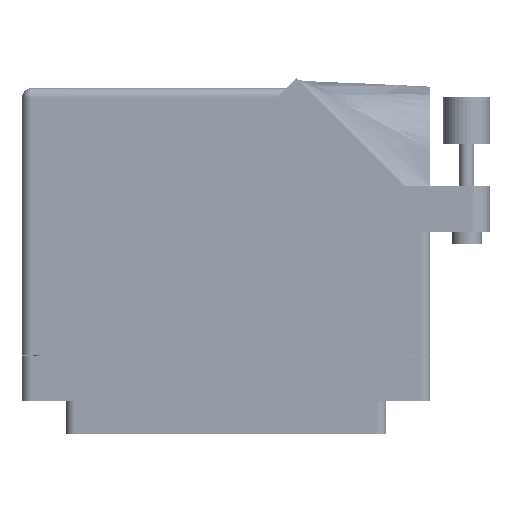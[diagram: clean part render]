
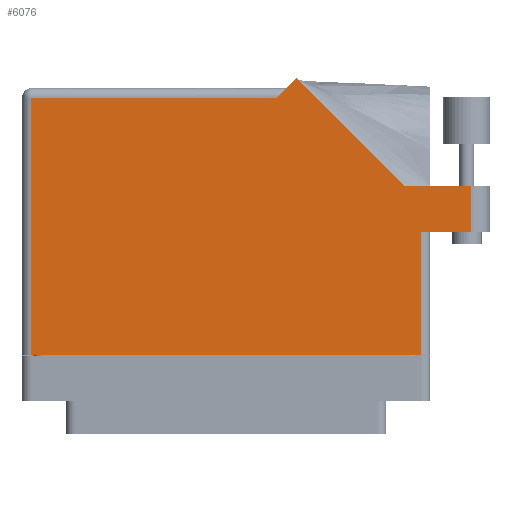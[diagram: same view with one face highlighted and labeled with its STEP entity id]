
A CAD part, front view. The second image highlights one B-rep face of the part: STEP entity #6076.
In plain terms, the highlighted face is planar.
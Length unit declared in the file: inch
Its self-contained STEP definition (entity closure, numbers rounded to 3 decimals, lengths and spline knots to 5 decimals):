
#868 = CARTESIAN_POINT ( 'NONE',  ( 1.359, 0.715, 0.617 ) ) ;
#1662 = VERTEX_POINT ( 'NONE', #10121 ) ;
#1802 = VERTEX_POINT ( 'NONE', #48628 ) ;
#1908 = VECTOR ( 'NONE', #8769, 39.37008 ) ;
#2494 = DIRECTION ( 'NONE',  ( 0., 1., 0. ) ) ;
#3832 = VECTOR ( 'NONE', #12226, 39.37008 ) ;
#4876 = CARTESIAN_POINT ( 'NONE',  ( -1.359, 1.613, 0.617 ) ) ;
#5480 = ORIENTED_EDGE ( 'NONE', *, *, #29514, .T. ) ;
#5575 = CARTESIAN_POINT ( 'NONE',  ( 1.297, 0.715, 0.617 ) ) ;
#6076 = ADVANCED_FACE ( 'NONE', ( #17635 ), #61496, .F. ) ;
#6463 = EDGE_CURVE ( 'NONE', #30711, #50482, #65937, .T. ) ;
#7562 = CARTESIAN_POINT ( 'NONE',  ( 1.297, 0.715, 0.617 ) ) ;
#8769 = DIRECTION ( 'NONE',  ( 0., 1., 0. ) ) ;
#8822 = CARTESIAN_POINT ( 'NONE',  ( 1.634, 1.022, 0.617 ) ) ;
#9809 = ORIENTED_EDGE ( 'NONE', *, *, #14939, .T. ) ;
#10024 = EDGE_CURVE ( 'NONE', #1802, #54385, #40155, .T. ) ;
#10121 = CARTESIAN_POINT ( 'NONE',  ( 0.46971, 1.74571, 0.617 ) ) ;
#10816 = CARTESIAN_POINT ( 'NONE',  ( 0.399, 1.675, 0.617 ) ) ;
#11078 = DIRECTION ( 'NONE',  ( -1., 0., 0. ) ) ;
#11191 = VECTOR ( 'NONE', #18649, 39.37008 ) ;
#12226 = DIRECTION ( 'NONE',  ( -0.707, 0.707, 0. ) ) ;
#14412 = VERTEX_POINT ( 'NONE', #29894 ) ;
#14939 = EDGE_CURVE ( 'NONE', #50482, #19580, #47428, .T. ) ;
#16135 = VECTOR ( 'NONE', #55921, 39.37008 ) ;
#17635 = FACE_OUTER_BOUND ( 'NONE', #51609, .T. ) ;
#18326 = LINE ( 'NONE', #22954, #3832 ) ;
#18385 = EDGE_CURVE ( 'NONE', #54385, #14412, #27615, .T. ) ;
#18621 = CARTESIAN_POINT ( 'NONE',  ( 1.759, 1.022, 0.617 ) ) ;
#18649 = DIRECTION ( 'NONE',  ( 0., -1., 0. ) ) ;
#19580 = VERTEX_POINT ( 'NONE', #8822 ) ;
#20605 = DIRECTION ( 'NONE',  ( 1., 0., 0. ) ) ;
#22954 = CARTESIAN_POINT ( 'NONE',  ( 1.19342, 1.022, 0.617 ) ) ;
#25347 = LINE ( 'NONE', #18621, #67749 ) ;
#26410 = LINE ( 'NONE', #4876, #32932 ) ;
#26836 = ORIENTED_EDGE ( 'NONE', *, *, #67394, .T. ) ;
#27278 = EDGE_CURVE ( 'NONE', #14412, #30711, #47818, .T. ) ;
#27615 = LINE ( 'NONE', #60590, #53027 ) ;
#29134 = CARTESIAN_POINT ( 'NONE',  ( -1.297, -0.1, 0.617 ) ) ;
#29514 = EDGE_CURVE ( 'NONE', #1662, #36642, #34059, .T. ) ;
#29646 = CARTESIAN_POINT ( 'NONE',  ( 1.634, 1.022, 0.617 ) ) ;
#29894 = CARTESIAN_POINT ( 'NONE',  ( 1.297, -0.1, 0.617 ) ) ;
#30711 = VERTEX_POINT ( 'NONE', #5575 ) ;
#32504 = ORIENTED_EDGE ( 'NONE', *, *, #41628, .T. ) ;
#32932 = VECTOR ( 'NONE', #11078, 39.37008 ) ;
#34059 = LINE ( 'NONE', #10816, #16135 ) ;
#34781 = EDGE_CURVE ( 'NONE', #64329, #1662, #18326, .T. ) ;
#35302 = DIRECTION ( 'NONE',  ( -1., 0., 0. ) ) ;
#36444 = DIRECTION ( 'NONE',  ( -1., 0., 0. ) ) ;
#36489 = ORIENTED_EDGE ( 'NONE', *, *, #10024, .T. ) ;
#36642 = VERTEX_POINT ( 'NONE', #54017 ) ;
#37693 = CARTESIAN_POINT ( 'NONE',  ( -1.297, -0.1, 0.617 ) ) ;
#38258 = CARTESIAN_POINT ( 'NONE',  ( 1.634, 0.715, 0.617 ) ) ;
#38642 = ORIENTED_EDGE ( 'NONE', *, *, #18385, .T. ) ;
#40155 = LINE ( 'NONE', #29134, #11191 ) ;
#40264 = CARTESIAN_POINT ( 'NONE',  ( -1.359, 1.675, 0.617 ) ) ;
#40407 = ORIENTED_EDGE ( 'NONE', *, *, #27278, .T. ) ;
#41628 = EDGE_CURVE ( 'NONE', #19580, #64329, #25347, .T. ) ;
#43174 = DIRECTION ( 'NONE',  ( 1., 0., 0. ) ) ;
#47428 = LINE ( 'NONE', #29646, #62671 ) ;
#47818 = LINE ( 'NONE', #7562, #1908 ) ;
#48628 = CARTESIAN_POINT ( 'NONE',  ( -1.297, 1.613, 0.617 ) ) ;
#50482 = VERTEX_POINT ( 'NONE', #38258 ) ;
#51585 = VECTOR ( 'NONE', #43174, 39.37008 ) ;
#51597 = DIRECTION ( 'NONE',  ( 0., 0., -1. ) ) ;
#51609 = EDGE_LOOP ( 'NONE', ( #55543, #9809, #32504, #52272, #5480, #26836, #36489, #38642, #40407 ) ) ;
#52272 = ORIENTED_EDGE ( 'NONE', *, *, #34781, .T. ) ;
#53027 = VECTOR ( 'NONE', #20605, 39.37008 ) ;
#54017 = CARTESIAN_POINT ( 'NONE',  ( 0.337, 1.613, 0.617 ) ) ;
#54385 = VERTEX_POINT ( 'NONE', #37693 ) ;
#55543 = ORIENTED_EDGE ( 'NONE', *, *, #6463, .T. ) ;
#55921 = DIRECTION ( 'NONE',  ( -0.707, -0.707, 0. ) ) ;
#60590 = CARTESIAN_POINT ( 'NONE',  ( -1.359, -0.1, 0.617 ) ) ;
#61496 = PLANE ( 'NONE',  #63625 ) ;
#62671 = VECTOR ( 'NONE', #2494, 39.37008 ) ;
#63625 = AXIS2_PLACEMENT_3D ( 'NONE', #40264, #51597, #36444 ) ;
#64329 = VERTEX_POINT ( 'NONE', #67327 ) ;
#65937 = LINE ( 'NONE', #868, #51585 ) ;
#67327 = CARTESIAN_POINT ( 'NONE',  ( 1.19342, 1.022, 0.617 ) ) ;
#67394 = EDGE_CURVE ( 'NONE', #36642, #1802, #26410, .T. ) ;
#67749 = VECTOR ( 'NONE', #35302, 39.37008 ) ;
